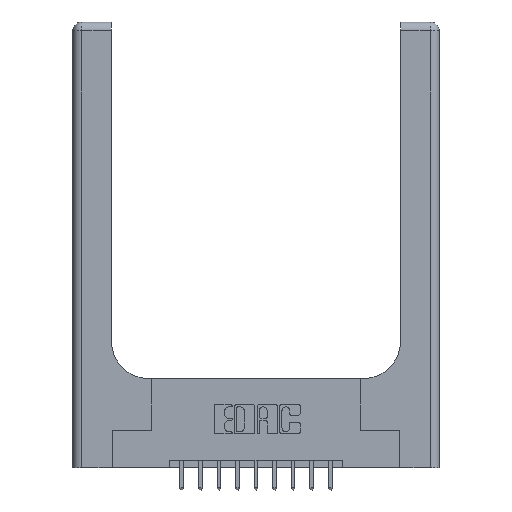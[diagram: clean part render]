
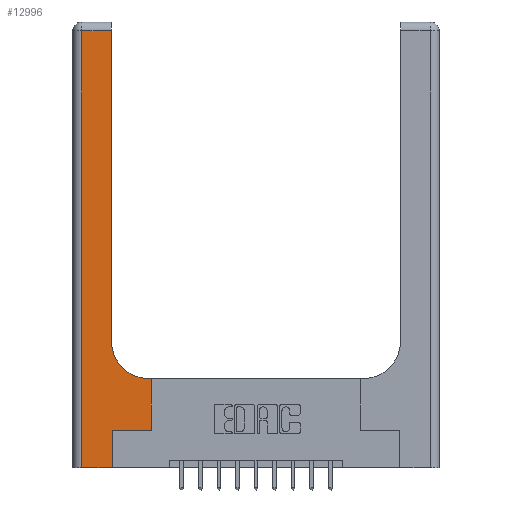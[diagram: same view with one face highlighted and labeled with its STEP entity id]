
A CAD part, top view. The second image highlights one B-rep face of the part: STEP entity #12996.
In plain terms, the highlighted planar face has unit normal (0, 0, 1).
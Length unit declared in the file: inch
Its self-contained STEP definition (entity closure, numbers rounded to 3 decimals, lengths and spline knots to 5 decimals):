
#13 = LINE ( 'NONE', #13540, #5392 ) ;
#216 = EDGE_LOOP ( 'NONE', ( #7037, #1251, #5538, #5053, #499, #11227, #13746, #15446, #3505 ) ) ;
#252 = CARTESIAN_POINT ( 'NONE',  ( 0.528, 0.6, 0.37 ) ) ;
#499 = ORIENTED_EDGE ( 'NONE', *, *, #13400, .T. ) ;
#602 = VECTOR ( 'NONE', #4378, 39.37008 ) ;
#669 = LINE ( 'NONE', #14253, #602 ) ;
#1251 = ORIENTED_EDGE ( 'NONE', *, *, #8362, .T. ) ;
#1468 = AXIS2_PLACEMENT_3D ( 'NONE', #8567, #9768, #7099 ) ;
#1604 = CARTESIAN_POINT ( 'NONE',  ( 0.528, 0.25, 0.37 ) ) ;
#1624 = DIRECTION ( 'NONE',  ( 0., 1., 0. ) ) ;
#1714 = VERTEX_POINT ( 'NONE', #8556 ) ;
#1886 = DIRECTION ( 'NONE',  ( 0., 1., 0. ) ) ;
#2103 = VECTOR ( 'NONE', #9609, 39.37008 ) ;
#2423 = LINE ( 'NONE', #4841, #7166 ) ;
#2494 = CARTESIAN_POINT ( 'NONE',  ( 0.26, 0.6, 0.37 ) ) ;
#2584 = VERTEX_POINT ( 'NONE', #252 ) ;
#2788 = CARTESIAN_POINT ( 'NONE',  ( 0., 0., 0.37 ) ) ;
#3505 = ORIENTED_EDGE ( 'NONE', *, *, #6429, .T. ) ;
#3602 = DIRECTION ( 'NONE',  ( 0., 1., 0. ) ) ;
#3890 = VECTOR ( 'NONE', #1886, 39.37008 ) ;
#3936 = DIRECTION ( 'NONE',  ( 1., 0., 0. ) ) ;
#4050 = CARTESIAN_POINT ( 'NONE',  ( 0.528, 0.25, 0.37 ) ) ;
#4081 = LINE ( 'NONE', #6742, #3890 ) ;
#4120 = EDGE_CURVE ( 'NONE', #14979, #5217, #11487, .T. ) ;
#4145 = CARTESIAN_POINT ( 'NONE',  ( 0.51, 0.6, 0.37 ) ) ;
#4378 = DIRECTION ( 'NONE',  ( 0., -1., 0. ) ) ;
#4574 = EDGE_CURVE ( 'NONE', #6169, #2584, #6476, .T. ) ;
#4841 = CARTESIAN_POINT ( 'NONE',  ( 0.265, 0.25, 0.37 ) ) ;
#5053 = ORIENTED_EDGE ( 'NONE', *, *, #4120, .T. ) ;
#5217 = VERTEX_POINT ( 'NONE', #12239 ) ;
#5392 = VECTOR ( 'NONE', #3602, 39.37008 ) ;
#5538 = ORIENTED_EDGE ( 'NONE', *, *, #9922, .T. ) ;
#5570 = VERTEX_POINT ( 'NONE', #15802 ) ;
#5725 = DIRECTION ( 'NONE',  ( 0., 0., -1. ) ) ;
#5898 = PLANE ( 'NONE',  #15236 ) ;
#6022 = VERTEX_POINT ( 'NONE', #9697 ) ;
#6169 = VERTEX_POINT ( 'NONE', #1604 ) ;
#6429 = EDGE_CURVE ( 'NONE', #15390, #1714, #7680, .T. ) ;
#6476 = LINE ( 'NONE', #4050, #15660 ) ;
#6742 = CARTESIAN_POINT ( 'NONE',  ( 0.26, 3., 0.37 ) ) ;
#7037 = ORIENTED_EDGE ( 'NONE', *, *, #7132, .T. ) ;
#7099 = DIRECTION ( 'NONE',  ( 1., 0., 0. ) ) ;
#7132 = EDGE_CURVE ( 'NONE', #1714, #6022, #4081, .T. ) ;
#7166 = VECTOR ( 'NONE', #3936, 39.37008 ) ;
#7680 = CIRCLE ( 'NONE', #1468, 0.25 ) ;
#7745 = VECTOR ( 'NONE', #14095, 39.37008 ) ;
#7914 = EDGE_CURVE ( 'NONE', #2584, #15390, #9853, .T. ) ;
#8219 = CARTESIAN_POINT ( 'NONE',  ( 0., 2.94, 0.37 ) ) ;
#8362 = EDGE_CURVE ( 'NONE', #6022, #5570, #14264, .T. ) ;
#8556 = CARTESIAN_POINT ( 'NONE',  ( 0.26, 0.85, 0.37 ) ) ;
#8567 = CARTESIAN_POINT ( 'NONE',  ( 0.51, 0.85, 0.37 ) ) ;
#9092 = VECTOR ( 'NONE', #9178, 39.37008 ) ;
#9178 = DIRECTION ( 'NONE',  ( -1., 0., 0. ) ) ;
#9239 = CARTESIAN_POINT ( 'NONE',  ( 0.06, 0., 0.37 ) ) ;
#9311 = CARTESIAN_POINT ( 'NONE',  ( 0.265, 0.25, 0.37 ) ) ;
#9609 = DIRECTION ( 'NONE',  ( -1., 0., 0. ) ) ;
#9697 = CARTESIAN_POINT ( 'NONE',  ( 0.26, 2.94, 0.37 ) ) ;
#9768 = DIRECTION ( 'NONE',  ( 0., 0., -1. ) ) ;
#9853 = LINE ( 'NONE', #2494, #2103 ) ;
#9922 = EDGE_CURVE ( 'NONE', #5570, #14979, #669, .T. ) ;
#10638 = DIRECTION ( 'NONE',  ( -1., 0., 0. ) ) ;
#11227 = ORIENTED_EDGE ( 'NONE', *, *, #14184, .T. ) ;
#11487 = LINE ( 'NONE', #2788, #7745 ) ;
#11866 = FACE_OUTER_BOUND ( 'NONE', #216, .T. ) ;
#12239 = CARTESIAN_POINT ( 'NONE',  ( 0.265, 0., 0.37 ) ) ;
#12996 = ADVANCED_FACE ( 'NONE', ( #11866 ), #5898, .F. ) ;
#13400 = EDGE_CURVE ( 'NONE', #5217, #15052, #13, .T. ) ;
#13540 = CARTESIAN_POINT ( 'NONE',  ( 0.265, 0., 0.37 ) ) ;
#13746 = ORIENTED_EDGE ( 'NONE', *, *, #4574, .T. ) ;
#14095 = DIRECTION ( 'NONE',  ( 1., 0., 0. ) ) ;
#14184 = EDGE_CURVE ( 'NONE', #15052, #6169, #2423, .T. ) ;
#14253 = CARTESIAN_POINT ( 'NONE',  ( 0.06, 3., 0.37 ) ) ;
#14264 = LINE ( 'NONE', #8219, #9092 ) ;
#14543 = CARTESIAN_POINT ( 'NONE',  ( 0., 3., 0.37 ) ) ;
#14979 = VERTEX_POINT ( 'NONE', #9239 ) ;
#15052 = VERTEX_POINT ( 'NONE', #9311 ) ;
#15236 = AXIS2_PLACEMENT_3D ( 'NONE', #14543, #5725, #10638 ) ;
#15390 = VERTEX_POINT ( 'NONE', #4145 ) ;
#15446 = ORIENTED_EDGE ( 'NONE', *, *, #7914, .T. ) ;
#15660 = VECTOR ( 'NONE', #1624, 39.37008 ) ;
#15802 = CARTESIAN_POINT ( 'NONE',  ( 0.06, 2.94, 0.37 ) ) ;
